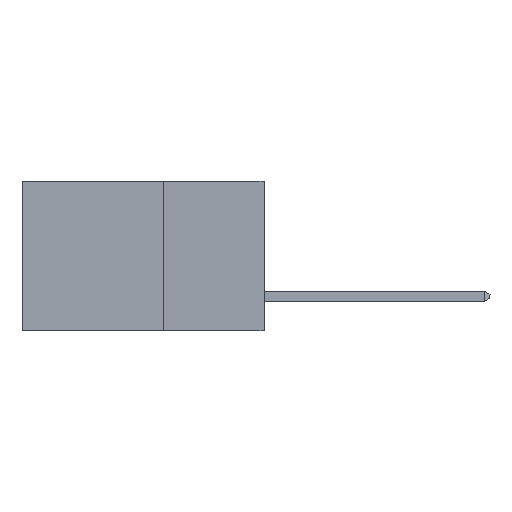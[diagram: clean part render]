
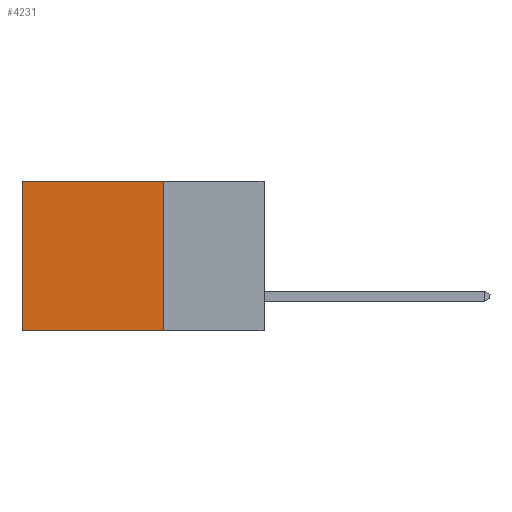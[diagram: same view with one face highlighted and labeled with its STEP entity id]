
A CAD part, left-side view. The second image highlights one B-rep face of the part: STEP entity #4231.
In plain terms, the highlighted planar face has unit normal (-1, 0, 0).
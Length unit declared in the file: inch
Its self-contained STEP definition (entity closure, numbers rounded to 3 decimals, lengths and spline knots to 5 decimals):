
#243 = LINE ( 'NONE', #908, #9046 ) ;
#641 = DIRECTION ( 'NONE',  ( 1., 0., 0. ) ) ;
#790 = ORIENTED_EDGE ( 'NONE', *, *, #2003, .F. ) ;
#908 = CARTESIAN_POINT ( 'NONE',  ( 0.2615, 0.25, 0. ) ) ;
#1454 = VERTEX_POINT ( 'NONE', #3813 ) ;
#1540 = CARTESIAN_POINT ( 'NONE',  ( 0.2615, 0.6, 0. ) ) ;
#1714 = EDGE_LOOP ( 'NONE', ( #9914, #8931, #790, #8515 ) ) ;
#1850 = VERTEX_POINT ( 'NONE', #1540 ) ;
#2003 = EDGE_CURVE ( 'NONE', #5864, #3339, #9647, .T. ) ;
#2966 = LINE ( 'NONE', #4351, #8651 ) ;
#3249 = CARTESIAN_POINT ( 'NONE',  ( 0.2615, 0.25, -0.37 ) ) ;
#3339 = VERTEX_POINT ( 'NONE', #7092 ) ;
#3429 = DIRECTION ( 'NONE',  ( 0., 0., -1. ) ) ;
#3813 = CARTESIAN_POINT ( 'NONE',  ( 0.2615, 0.6, -0.37 ) ) ;
#4231 = ADVANCED_FACE ( 'NONE', ( #4516 ), #9724, .F. ) ;
#4351 = CARTESIAN_POINT ( 'NONE',  ( 0.2615, 0.6, -0.37 ) ) ;
#4516 = FACE_OUTER_BOUND ( 'NONE', #1714, .T. ) ;
#4578 = EDGE_CURVE ( 'NONE', #1850, #1454, #2966, .T. ) ;
#4648 = VECTOR ( 'NONE', #10025, 39.37008 ) ;
#4767 = LINE ( 'NONE', #3249, #4648 ) ;
#5195 = EDGE_CURVE ( 'NONE', #3339, #1454, #4767, .T. ) ;
#5426 = VECTOR ( 'NONE', #3429, 39.37008 ) ;
#5864 = VERTEX_POINT ( 'NONE', #6519 ) ;
#5984 = DIRECTION ( 'NONE',  ( 0., 0., -1. ) ) ;
#6075 = CARTESIAN_POINT ( 'NONE',  ( 0.2615, 0.25, -0.37 ) ) ;
#6225 = AXIS2_PLACEMENT_3D ( 'NONE', #6075, #641, #5984 ) ;
#6519 = CARTESIAN_POINT ( 'NONE',  ( 0.2615, 0.25, 0. ) ) ;
#7092 = CARTESIAN_POINT ( 'NONE',  ( 0.2615, 0.25, -0.37 ) ) ;
#7938 = CARTESIAN_POINT ( 'NONE',  ( 0.2615, 0.25, -0.37 ) ) ;
#8016 = DIRECTION ( 'NONE',  ( 0., 1., 0. ) ) ;
#8515 = ORIENTED_EDGE ( 'NONE', *, *, #9798, .T. ) ;
#8651 = VECTOR ( 'NONE', #9859, 39.37008 ) ;
#8931 = ORIENTED_EDGE ( 'NONE', *, *, #5195, .F. ) ;
#9046 = VECTOR ( 'NONE', #8016, 39.37008 ) ;
#9647 = LINE ( 'NONE', #7938, #5426 ) ;
#9724 = PLANE ( 'NONE',  #6225 ) ;
#9798 = EDGE_CURVE ( 'NONE', #5864, #1850, #243, .T. ) ;
#9859 = DIRECTION ( 'NONE',  ( 0., 0., -1. ) ) ;
#9914 = ORIENTED_EDGE ( 'NONE', *, *, #4578, .T. ) ;
#10025 = DIRECTION ( 'NONE',  ( 0., 1., 0. ) ) ;
